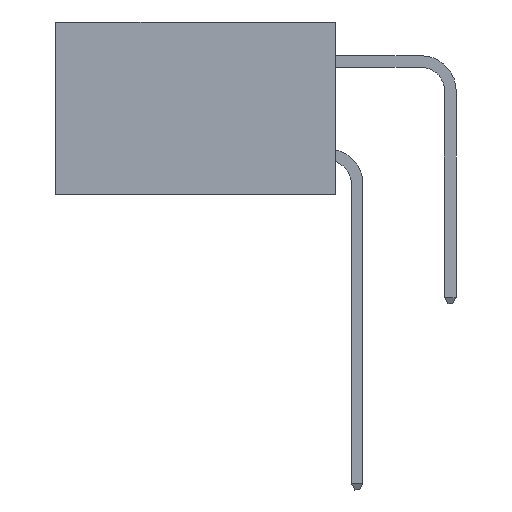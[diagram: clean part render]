
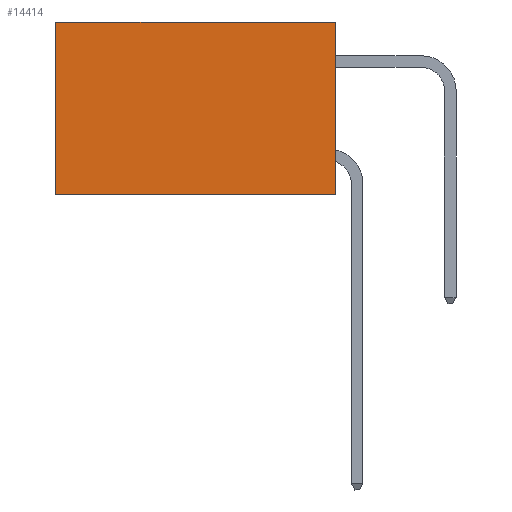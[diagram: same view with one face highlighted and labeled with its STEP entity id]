
A CAD part, left-side view. The second image highlights one B-rep face of the part: STEP entity #14414.
In plain terms, the highlighted planar face has unit normal (-1, 0, 0).
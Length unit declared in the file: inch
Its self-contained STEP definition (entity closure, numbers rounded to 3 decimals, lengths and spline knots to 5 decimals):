
#1069 = ORIENTED_EDGE ( 'NONE', *, *, #14180, .F. ) ;
#2186 = PLANE ( 'NONE',  #14676 ) ;
#2193 = LINE ( 'NONE', #20215, #11530 ) ;
#2301 = CARTESIAN_POINT ( 'NONE',  ( 0.2875, 0.6, 0. ) ) ;
#3496 = CARTESIAN_POINT ( 'NONE',  ( 0.2875, 0., 0. ) ) ;
#4061 = DIRECTION ( 'NONE',  ( 1., 0., 0. ) ) ;
#4088 = VECTOR ( 'NONE', #7478, 39.37008 ) ;
#4867 = VECTOR ( 'NONE', #5311, 39.37008 ) ;
#4956 = ORIENTED_EDGE ( 'NONE', *, *, #8675, .F. ) ;
#5311 = DIRECTION ( 'NONE',  ( 0., 0., -1. ) ) ;
#5363 = VECTOR ( 'NONE', #19506, 39.37008 ) ;
#5502 = DIRECTION ( 'NONE',  ( 0., 1., 0. ) ) ;
#5672 = VERTEX_POINT ( 'NONE', #6181 ) ;
#6181 = CARTESIAN_POINT ( 'NONE',  ( 0.2875, 0., -0.37 ) ) ;
#7478 = DIRECTION ( 'NONE',  ( 0., 1., 0. ) ) ;
#8675 = EDGE_CURVE ( 'NONE', #16355, #5672, #19638, .T. ) ;
#8966 = LINE ( 'NONE', #16703, #4088 ) ;
#10989 = ORIENTED_EDGE ( 'NONE', *, *, #22343, .T. ) ;
#11530 = VECTOR ( 'NONE', #5502, 39.37008 ) ;
#11785 = VERTEX_POINT ( 'NONE', #2301 ) ;
#12271 = CARTESIAN_POINT ( 'NONE',  ( 0.2875, 0.6, -0.37 ) ) ;
#14180 = EDGE_CURVE ( 'NONE', #5672, #20057, #8966, .T. ) ;
#14414 = ADVANCED_FACE ( 'NONE', ( #19112 ), #2186, .F. ) ;
#14676 = AXIS2_PLACEMENT_3D ( 'NONE', #15184, #4061, #17019 ) ;
#15184 = CARTESIAN_POINT ( 'NONE',  ( 0.2875, 0., 0. ) ) ;
#16355 = VERTEX_POINT ( 'NONE', #20514 ) ;
#16703 = CARTESIAN_POINT ( 'NONE',  ( 0.2875, 0., -0.37 ) ) ;
#17019 = DIRECTION ( 'NONE',  ( 0., 0., -1. ) ) ;
#17533 = EDGE_CURVE ( 'NONE', #11785, #20057, #20119, .T. ) ;
#17676 = CARTESIAN_POINT ( 'NONE',  ( 0.2875, 0.6, 0. ) ) ;
#19112 = FACE_OUTER_BOUND ( 'NONE', #23332, .T. ) ;
#19506 = DIRECTION ( 'NONE',  ( 0., 0., -1. ) ) ;
#19638 = LINE ( 'NONE', #3496, #4867 ) ;
#20057 = VERTEX_POINT ( 'NONE', #12271 ) ;
#20119 = LINE ( 'NONE', #17676, #5363 ) ;
#20215 = CARTESIAN_POINT ( 'NONE',  ( 0.2875, 0., 0. ) ) ;
#20514 = CARTESIAN_POINT ( 'NONE',  ( 0.2875, 0., 0. ) ) ;
#22343 = EDGE_CURVE ( 'NONE', #16355, #11785, #2193, .T. ) ;
#22490 = ORIENTED_EDGE ( 'NONE', *, *, #17533, .T. ) ;
#23332 = EDGE_LOOP ( 'NONE', ( #22490, #1069, #4956, #10989 ) ) ;
